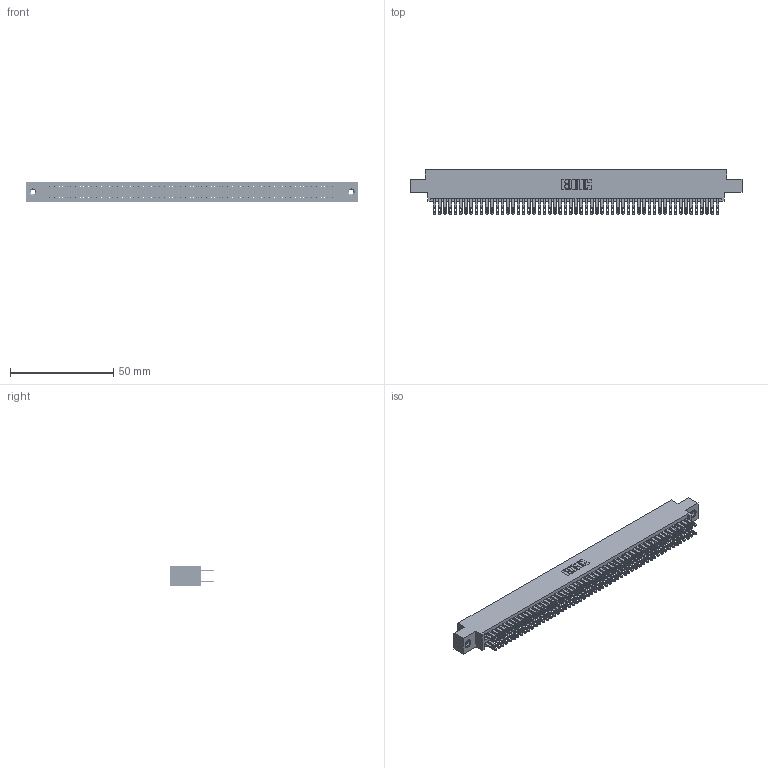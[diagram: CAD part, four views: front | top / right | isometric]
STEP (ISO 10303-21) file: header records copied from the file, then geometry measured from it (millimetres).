
FILE_DESCRIPTION (( 'STEP AP203' ), '1' );
FILE_NAME ('345-110-500-808.STEP', '2018-10-07T08:54:19', ( '' ), ( '' ), 'SwSTEP 2.0', 'SolidWorks 2016', '' );
FILE_SCHEMA (( 'CONFIG_CONTROL_DESIGN' ));
Length unit declared in the file: inch
Products named in the file (4): 345 Part_0.170 Offset - 0.156 Dia-TI; 345-250-001_345-250-003-102; 345-292-001_345-293-100; 345-110-500-808
Assembly tree (113 placements, depth 2):
  345-110-500-808
    345 Part_0.170 Offset - 0.156 Dia-TI
    345-292-001_345-293-100  x110
    345-250-001_345-250-003-102  x2
Bounding box: 160.91 x 21.51 x 9.4 mm (x, y, z)
Volume: 15967.8 mm3; surface area: 25133.7 mm2
Topology: 113 solids, 113 shells, 5250 faces, 15999 edges, 10658 vertices
Faces by surface type: plane 3086, cylinder 2148, cone 12, torus 4
Entity records: 42652 total; most frequent: CARTESIAN_POINT 7119, ORIENTED_EDGE 7046, DIRECTION 6289, EDGE_CURVE 3523, LINE 3147, VECTOR 3147, VERTEX_POINT 2344, AXIS2_PLACEMENT_3D 1571
